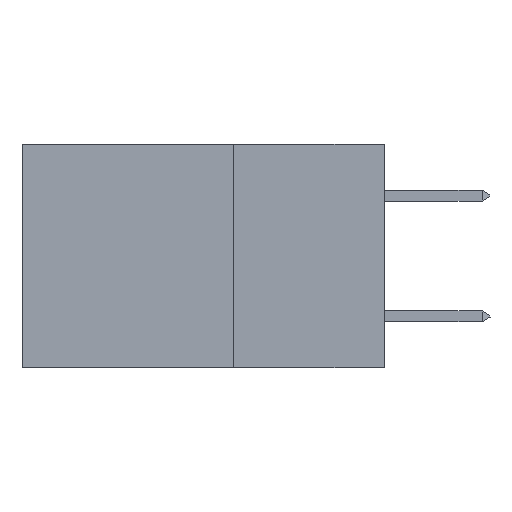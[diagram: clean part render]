
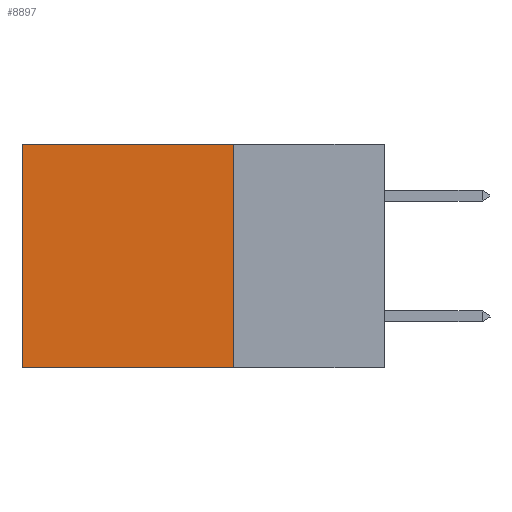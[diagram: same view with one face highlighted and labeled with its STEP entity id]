
A CAD part, left-side view. The second image highlights one B-rep face of the part: STEP entity #8897.
In plain terms, the highlighted planar face has unit normal (-1, 0, 0).
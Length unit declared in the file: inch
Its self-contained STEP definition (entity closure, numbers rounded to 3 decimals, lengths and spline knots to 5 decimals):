
#96 = VECTOR ( 'NONE', #7713, 39.37008 ) ;
#1277 = EDGE_CURVE ( 'NONE', #4603, #11134, #5058, .T. ) ;
#1640 = EDGE_CURVE ( 'NONE', #10691, #11134, #2006, .T. ) ;
#1705 = DIRECTION ( 'NONE',  ( 0., 0., -1. ) ) ;
#1883 = CARTESIAN_POINT ( 'NONE',  ( 0.2875, 0.6, 0. ) ) ;
#2006 = LINE ( 'NONE', #1883, #9252 ) ;
#2435 = CARTESIAN_POINT ( 'NONE',  ( 0.2875, 0.6, 0. ) ) ;
#2628 = CARTESIAN_POINT ( 'NONE',  ( 0.2875, 0.25, 0. ) ) ;
#2941 = ORIENTED_EDGE ( 'NONE', *, *, #1640, .T. ) ;
#4389 = DIRECTION ( 'NONE',  ( 0., 0., -1. ) ) ;
#4603 = VERTEX_POINT ( 'NONE', #10209 ) ;
#4902 = VECTOR ( 'NONE', #12103, 39.37008 ) ;
#4948 = ORIENTED_EDGE ( 'NONE', *, *, #10549, .T. ) ;
#5058 = LINE ( 'NONE', #7706, #96 ) ;
#5319 = CARTESIAN_POINT ( 'NONE',  ( 0.2875, 0.25, 0. ) ) ;
#5520 = LINE ( 'NONE', #11131, #4902 ) ;
#5832 = EDGE_CURVE ( 'NONE', #10665, #4603, #12266, .T. ) ;
#7022 = VECTOR ( 'NONE', #11492, 39.37008 ) ;
#7706 = CARTESIAN_POINT ( 'NONE',  ( 0.2875, 0.25, -0.37 ) ) ;
#7713 = DIRECTION ( 'NONE',  ( 0., 1., 0. ) ) ;
#8724 = CARTESIAN_POINT ( 'NONE',  ( 0.2875, 0.6, -0.37 ) ) ;
#8897 = ADVANCED_FACE ( 'NONE', ( #9129 ), #10307, .F. ) ;
#9129 = FACE_OUTER_BOUND ( 'NONE', #10672, .T. ) ;
#9252 = VECTOR ( 'NONE', #1705, 39.37008 ) ;
#9326 = CARTESIAN_POINT ( 'NONE',  ( 0.2875, 0.25, 0. ) ) ;
#10209 = CARTESIAN_POINT ( 'NONE',  ( 0.2875, 0.25, -0.37 ) ) ;
#10257 = DIRECTION ( 'NONE',  ( 1., 0., 0. ) ) ;
#10307 = PLANE ( 'NONE',  #11724 ) ;
#10358 = ORIENTED_EDGE ( 'NONE', *, *, #5832, .F. ) ;
#10549 = EDGE_CURVE ( 'NONE', #10665, #10691, #5520, .T. ) ;
#10665 = VERTEX_POINT ( 'NONE', #5319 ) ;
#10672 = EDGE_LOOP ( 'NONE', ( #2941, #11304, #10358, #4948 ) ) ;
#10691 = VERTEX_POINT ( 'NONE', #2435 ) ;
#11131 = CARTESIAN_POINT ( 'NONE',  ( 0.2875, 0.25, 0. ) ) ;
#11134 = VERTEX_POINT ( 'NONE', #8724 ) ;
#11304 = ORIENTED_EDGE ( 'NONE', *, *, #1277, .F. ) ;
#11492 = DIRECTION ( 'NONE',  ( 0., 0., -1. ) ) ;
#11724 = AXIS2_PLACEMENT_3D ( 'NONE', #9326, #10257, #4389 ) ;
#12103 = DIRECTION ( 'NONE',  ( 0., 1., 0. ) ) ;
#12266 = LINE ( 'NONE', #2628, #7022 ) ;
